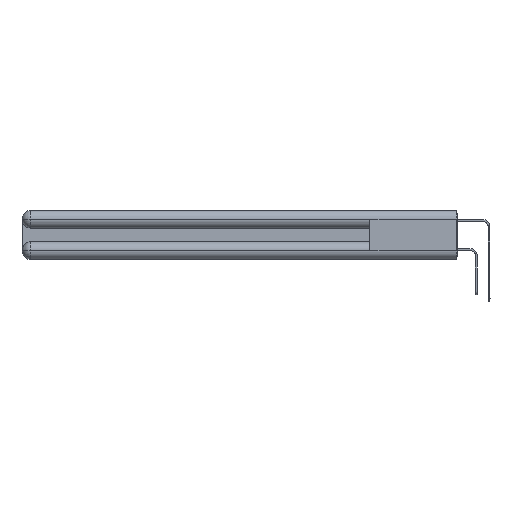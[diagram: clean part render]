
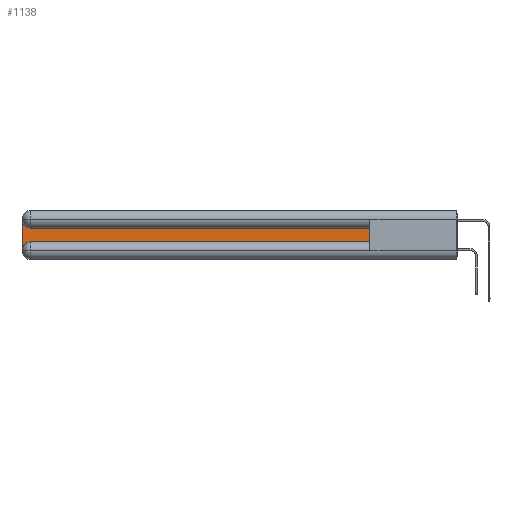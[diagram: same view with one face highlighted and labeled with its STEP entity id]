
A CAD part, left-side view. The second image highlights one B-rep face of the part: STEP entity #1138.
In plain terms, the highlighted planar face has unit normal (-1, 0, 0).
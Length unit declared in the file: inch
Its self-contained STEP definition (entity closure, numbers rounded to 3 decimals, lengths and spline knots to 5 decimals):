
#107 = VECTOR ( 'NONE', #3073, 39.37008 ) ;
#670 = DIRECTION ( 'NONE',  ( 1., 0., 0. ) ) ;
#865 = ORIENTED_EDGE ( 'NONE', *, *, #8336, .T. ) ;
#1138 = ADVANCED_FACE ( 'NONE', ( #27676 ), #16159, .F. ) ;
#1570 = CARTESIAN_POINT ( 'NONE',  ( 0.075, 2.94, -0.2775 ) ) ;
#2256 = CARTESIAN_POINT ( 'NONE',  ( 0.075, 0.6, -0.1225 ) ) ;
#3073 = DIRECTION ( 'NONE',  ( 0., 0., 1. ) ) ;
#3428 = CARTESIAN_POINT ( 'NONE',  ( 0.075, 3., -0.1225 ) ) ;
#3584 = CIRCLE ( 'NONE', #11865, 0.06 ) ;
#3984 = CARTESIAN_POINT ( 'NONE',  ( 0.075, 2.94, -0.1225 ) ) ;
#4319 = LINE ( 'NONE', #23074, #25050 ) ;
#4342 = VERTEX_POINT ( 'NONE', #3984 ) ;
#4535 = CARTESIAN_POINT ( 'NONE',  ( 0.075, 0.6, -0.1225 ) ) ;
#4942 = EDGE_CURVE ( 'NONE', #22109, #4342, #13467, .T. ) ;
#4987 = DIRECTION ( 'NONE',  ( 0., 0., -1. ) ) ;
#6082 = ORIENTED_EDGE ( 'NONE', *, *, #8425, .T. ) ;
#6354 = ORIENTED_EDGE ( 'NONE', *, *, #13795, .T. ) ;
#6890 = CARTESIAN_POINT ( 'NONE',  ( 0.075, 0.6, -0.2175 ) ) ;
#7211 = LINE ( 'NONE', #7785, #17014 ) ;
#7257 = DIRECTION ( 'NONE',  ( 1., 0., 0. ) ) ;
#7785 = CARTESIAN_POINT ( 'NONE',  ( 0.075, 3., -0.2175 ) ) ;
#8336 = EDGE_CURVE ( 'NONE', #12701, #15726, #7211, .T. ) ;
#8425 = EDGE_CURVE ( 'NONE', #29499, #22109, #14017, .T. ) ;
#10100 = DIRECTION ( 'NONE',  ( 0., 0., -1. ) ) ;
#11654 = CARTESIAN_POINT ( 'NONE',  ( 0.075, 2.94, -0.0625 ) ) ;
#11865 = AXIS2_PLACEMENT_3D ( 'NONE', #11654, #7257, #4987 ) ;
#12285 = VECTOR ( 'NONE', #16192, 39.37008 ) ;
#12701 = VERTEX_POINT ( 'NONE', #14584 ) ;
#13467 = LINE ( 'NONE', #2256, #12285 ) ;
#13795 = EDGE_CURVE ( 'NONE', #15726, #27665, #28855, .T. ) ;
#14017 = LINE ( 'NONE', #23264, #107 ) ;
#14584 = CARTESIAN_POINT ( 'NONE',  ( 0.075, 3., -0.0625 ) ) ;
#15726 = VERTEX_POINT ( 'NONE', #26578 ) ;
#16159 = PLANE ( 'NONE',  #24902 ) ;
#16189 = CARTESIAN_POINT ( 'NONE',  ( 0.075, 2.94, -0.2175 ) ) ;
#16192 = DIRECTION ( 'NONE',  ( 0., 1., 0. ) ) ;
#17014 = VECTOR ( 'NONE', #17020, 39.37008 ) ;
#17020 = DIRECTION ( 'NONE',  ( 0., 0., -1. ) ) ;
#17254 = EDGE_CURVE ( 'NONE', #27665, #29499, #4319, .T. ) ;
#19612 = DIRECTION ( 'NONE',  ( 0., 0., -1. ) ) ;
#20062 = DIRECTION ( 'NONE',  ( 1., 0., 0. ) ) ;
#20809 = DIRECTION ( 'NONE',  ( 0., -1., 0. ) ) ;
#21933 = ORIENTED_EDGE ( 'NONE', *, *, #23375, .T. ) ;
#22109 = VERTEX_POINT ( 'NONE', #4535 ) ;
#22369 = ORIENTED_EDGE ( 'NONE', *, *, #4942, .T. ) ;
#23074 = CARTESIAN_POINT ( 'NONE',  ( 0.075, 0.6, -0.2175 ) ) ;
#23264 = CARTESIAN_POINT ( 'NONE',  ( 0.075, 0.6, -0.2175 ) ) ;
#23375 = EDGE_CURVE ( 'NONE', #4342, #12701, #3584, .T. ) ;
#24116 = EDGE_LOOP ( 'NONE', ( #22369, #21933, #865, #6354, #29301, #6082 ) ) ;
#24902 = AXIS2_PLACEMENT_3D ( 'NONE', #3428, #670, #10100 ) ;
#25050 = VECTOR ( 'NONE', #20809, 39.37008 ) ;
#25454 = AXIS2_PLACEMENT_3D ( 'NONE', #1570, #20062, #19612 ) ;
#26578 = CARTESIAN_POINT ( 'NONE',  ( 0.075, 3., -0.2775 ) ) ;
#27665 = VERTEX_POINT ( 'NONE', #16189 ) ;
#27676 = FACE_OUTER_BOUND ( 'NONE', #24116, .T. ) ;
#28855 = CIRCLE ( 'NONE', #25454, 0.06 ) ;
#29301 = ORIENTED_EDGE ( 'NONE', *, *, #17254, .T. ) ;
#29499 = VERTEX_POINT ( 'NONE', #6890 ) ;
